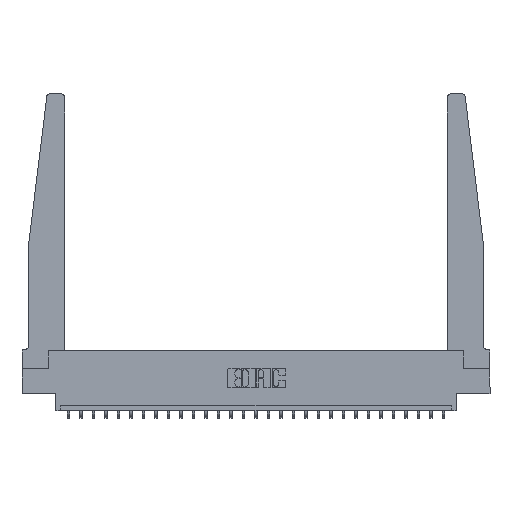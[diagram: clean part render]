
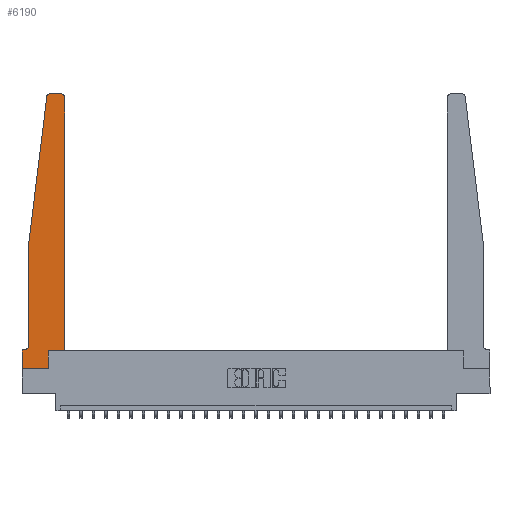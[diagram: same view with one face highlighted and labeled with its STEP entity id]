
A CAD part, top view. The second image highlights one B-rep face of the part: STEP entity #6190.
In plain terms, the highlighted planar face has unit normal (0, 0, 1).
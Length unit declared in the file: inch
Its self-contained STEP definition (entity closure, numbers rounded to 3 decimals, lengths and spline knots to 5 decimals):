
#68 = VERTEX_POINT ( 'NONE', #18164 ) ;
#526 = DIRECTION ( 'NONE',  ( 1., 0., 0. ) ) ;
#762 = VECTOR ( 'NONE', #10667, 39.37008 ) ;
#1093 = CARTESIAN_POINT ( 'NONE',  ( 0., 0., 0.37 ) ) ;
#1105 = LINE ( 'NONE', #8115, #16856 ) ;
#1218 = PLANE ( 'NONE',  #16150 ) ;
#1246 = CARTESIAN_POINT ( 'NONE',  ( 0.27653, 2.72, 0.37 ) ) ;
#1371 = CARTESIAN_POINT ( 'NONE',  ( 0.065, 0.2375, 0.37 ) ) ;
#1389 = LINE ( 'NONE', #4725, #762 ) ;
#1746 = CARTESIAN_POINT ( 'NONE',  ( 0.425, 0.18, 0.37 ) ) ;
#1937 = ORIENTED_EDGE ( 'NONE', *, *, #10923, .T. ) ;
#1986 = CARTESIAN_POINT ( 'NONE',  ( 0.425, 2.72, 0.37 ) ) ;
#1989 = DIRECTION ( 'NONE',  ( 0., 1., 0. ) ) ;
#2636 = EDGE_LOOP ( 'NONE', ( #12556, #13826, #1937, #4616, #21858, #21387, #14284, #19435, #12453, #19636, #9938, #19209 ) ) ;
#2645 = AXIS2_PLACEMENT_3D ( 'NONE', #24288, #12292, #526 ) ;
#3208 = DIRECTION ( 'NONE',  ( 1., 0., 0. ) ) ;
#3231 = DIRECTION ( 'NONE',  ( 1., 0., 0. ) ) ;
#3309 = CIRCLE ( 'NONE', #17430, 0.05 ) ;
#3919 = LINE ( 'NONE', #5719, #25079 ) ;
#4082 = EDGE_CURVE ( 'NONE', #5208, #13013, #16630, .T. ) ;
#4309 = VERTEX_POINT ( 'NONE', #1986 ) ;
#4384 = AXIS2_PLACEMENT_3D ( 'NONE', #1246, #15049, #3231 ) ;
#4616 = ORIENTED_EDGE ( 'NONE', *, *, #23290, .T. ) ;
#4717 = VERTEX_POINT ( 'NONE', #1371 ) ;
#4725 = CARTESIAN_POINT ( 'NONE',  ( 0.065, 1.25, 0.37 ) ) ;
#5208 = VERTEX_POINT ( 'NONE', #1093 ) ;
#5719 = CARTESIAN_POINT ( 'NONE',  ( 0., 0., 0.37 ) ) ;
#5858 = CARTESIAN_POINT ( 'NONE',  ( 0.065, 0.1875, 0.37 ) ) ;
#6190 = ADVANCED_FACE ( 'NONE', ( #17673 ), #1218, .T. ) ;
#6759 = CARTESIAN_POINT ( 'NONE',  ( 0., 0.1875, 0.37 ) ) ;
#7047 = DIRECTION ( 'NONE',  ( 1., 0., 0. ) ) ;
#7433 = EDGE_CURVE ( 'NONE', #17121, #19942, #16039, .T. ) ;
#7791 = LINE ( 'NONE', #21799, #23114 ) ;
#8115 = CARTESIAN_POINT ( 'NONE',  ( 0.25, 2.75, 0.37 ) ) ;
#8149 = LINE ( 'NONE', #21688, #18120 ) ;
#8518 = CARTESIAN_POINT ( 'NONE',  ( 0.24675, 2.72367, 0.37 ) ) ;
#8673 = EDGE_CURVE ( 'NONE', #24021, #5208, #3919, .T. ) ;
#8916 = CARTESIAN_POINT ( 'NONE',  ( 0., 0.1875, 0.37 ) ) ;
#9211 = CARTESIAN_POINT ( 'NONE',  ( 0.2605, 0.18, 0.37 ) ) ;
#9630 = VECTOR ( 'NONE', #12149, 39.37008 ) ;
#9938 = ORIENTED_EDGE ( 'NONE', *, *, #11361, .T. ) ;
#10140 = CARTESIAN_POINT ( 'NONE',  ( 0.065, 1.25, 0.37 ) ) ;
#10554 = LINE ( 'NONE', #1746, #20622 ) ;
#10667 = DIRECTION ( 'NONE',  ( 0., -1., 0. ) ) ;
#10813 = EDGE_CURVE ( 'NONE', #22837, #24021, #22777, .T. ) ;
#10923 = EDGE_CURVE ( 'NONE', #19942, #68, #14925, .T. ) ;
#11255 = CARTESIAN_POINT ( 'NONE',  ( 0.27653, 2.75, 0.37 ) ) ;
#11361 = EDGE_CURVE ( 'NONE', #11401, #4309, #10554, .T. ) ;
#11401 = VERTEX_POINT ( 'NONE', #19689 ) ;
#11545 = CARTESIAN_POINT ( 'NONE',  ( 0.015, 0.2375, 0.37 ) ) ;
#12108 = VECTOR ( 'NONE', #19805, 39.37008 ) ;
#12149 = DIRECTION ( 'NONE',  ( -0.122, -0.992, 0. ) ) ;
#12292 = DIRECTION ( 'NONE',  ( 0., 0., 1. ) ) ;
#12453 = ORIENTED_EDGE ( 'NONE', *, *, #23700, .T. ) ;
#12556 = ORIENTED_EDGE ( 'NONE', *, *, #15393, .T. ) ;
#12700 = EDGE_CURVE ( 'NONE', #4309, #17765, #12900, .T. ) ;
#12900 = CIRCLE ( 'NONE', #2645, 0.03 ) ;
#13013 = VERTEX_POINT ( 'NONE', #19397 ) ;
#13563 = DIRECTION ( 'NONE',  ( -1., 0., 0. ) ) ;
#13674 = VERTEX_POINT ( 'NONE', #9211 ) ;
#13826 = ORIENTED_EDGE ( 'NONE', *, *, #7433, .T. ) ;
#14284 = ORIENTED_EDGE ( 'NONE', *, *, #8673, .T. ) ;
#14572 = EDGE_CURVE ( 'NONE', #4717, #22837, #3309, .T. ) ;
#14706 = CARTESIAN_POINT ( 'NONE',  ( 0.015, 0.1875, 0.37 ) ) ;
#14925 = LINE ( 'NONE', #10140, #9630 ) ;
#15022 = DIRECTION ( 'NONE',  ( 0., 0., 1. ) ) ;
#15049 = DIRECTION ( 'NONE',  ( 0., 0., 1. ) ) ;
#15393 = EDGE_CURVE ( 'NONE', #17765, #17121, #1105, .T. ) ;
#16039 = CIRCLE ( 'NONE', #4384, 0.03 ) ;
#16150 = AXIS2_PLACEMENT_3D ( 'NONE', #8916, #15022, #3208 ) ;
#16630 = LINE ( 'NONE', #16953, #21998 ) ;
#16856 = VECTOR ( 'NONE', #20093, 39.37008 ) ;
#16953 = CARTESIAN_POINT ( 'NONE',  ( 0., 0., 0.37 ) ) ;
#17121 = VERTEX_POINT ( 'NONE', #11255 ) ;
#17430 = AXIS2_PLACEMENT_3D ( 'NONE', #11545, #25550, #13563 ) ;
#17481 = DIRECTION ( 'NONE',  ( 0., 1., 0. ) ) ;
#17673 = FACE_OUTER_BOUND ( 'NONE', #2636, .T. ) ;
#17765 = VERTEX_POINT ( 'NONE', #19196 ) ;
#18120 = VECTOR ( 'NONE', #23672, 39.37008 ) ;
#18164 = CARTESIAN_POINT ( 'NONE',  ( 0.065, 1.25, 0.37 ) ) ;
#19196 = CARTESIAN_POINT ( 'NONE',  ( 0.395, 2.75, 0.37 ) ) ;
#19209 = ORIENTED_EDGE ( 'NONE', *, *, #12700, .T. ) ;
#19397 = CARTESIAN_POINT ( 'NONE',  ( 0.2605, 0., 0.37 ) ) ;
#19435 = ORIENTED_EDGE ( 'NONE', *, *, #4082, .T. ) ;
#19636 = ORIENTED_EDGE ( 'NONE', *, *, #22500, .T. ) ;
#19654 = DIRECTION ( 'NONE',  ( 0., -1., 0. ) ) ;
#19689 = CARTESIAN_POINT ( 'NONE',  ( 0.425, 0.18, 0.37 ) ) ;
#19805 = DIRECTION ( 'NONE',  ( -1., 0., 0. ) ) ;
#19942 = VERTEX_POINT ( 'NONE', #8518 ) ;
#20093 = DIRECTION ( 'NONE',  ( -1., 0., 0. ) ) ;
#20622 = VECTOR ( 'NONE', #17481, 39.37008 ) ;
#21387 = ORIENTED_EDGE ( 'NONE', *, *, #10813, .T. ) ;
#21688 = CARTESIAN_POINT ( 'NONE',  ( 0.425, 0.18, 0.37 ) ) ;
#21799 = CARTESIAN_POINT ( 'NONE',  ( 0.2605, 0.18, 0.37 ) ) ;
#21858 = ORIENTED_EDGE ( 'NONE', *, *, #14572, .T. ) ;
#21998 = VECTOR ( 'NONE', #7047, 39.37008 ) ;
#22500 = EDGE_CURVE ( 'NONE', #13674, #11401, #8149, .T. ) ;
#22777 = LINE ( 'NONE', #5858, #12108 ) ;
#22837 = VERTEX_POINT ( 'NONE', #14706 ) ;
#23114 = VECTOR ( 'NONE', #1989, 39.37008 ) ;
#23290 = EDGE_CURVE ( 'NONE', #68, #4717, #1389, .T. ) ;
#23672 = DIRECTION ( 'NONE',  ( 1., 0., 0. ) ) ;
#23700 = EDGE_CURVE ( 'NONE', #13013, #13674, #7791, .T. ) ;
#24021 = VERTEX_POINT ( 'NONE', #6759 ) ;
#24288 = CARTESIAN_POINT ( 'NONE',  ( 0.395, 2.72, 0.37 ) ) ;
#25079 = VECTOR ( 'NONE', #19654, 39.37008 ) ;
#25550 = DIRECTION ( 'NONE',  ( 0., 0., -1. ) ) ;
